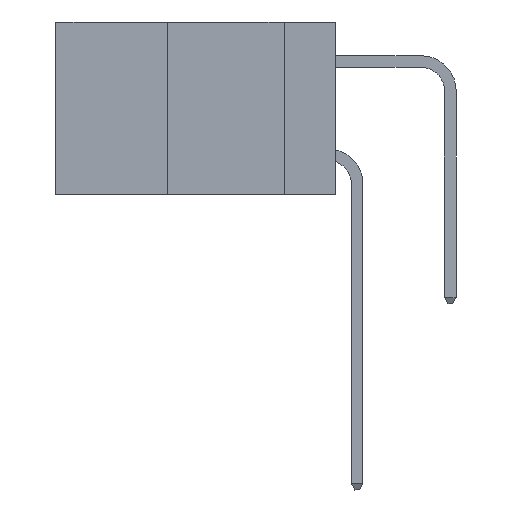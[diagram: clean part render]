
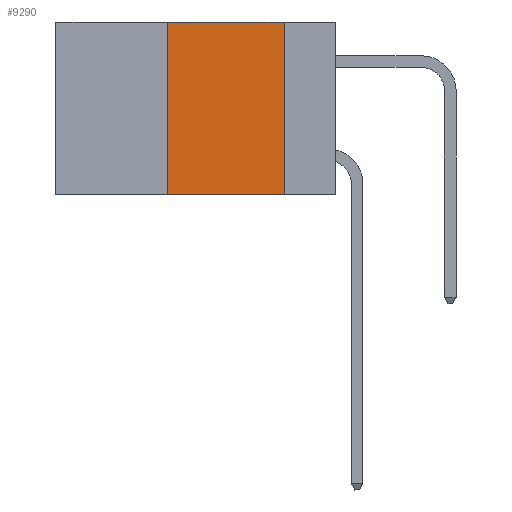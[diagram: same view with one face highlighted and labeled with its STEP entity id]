
A CAD part, left-side view. The second image highlights one B-rep face of the part: STEP entity #9290.
In plain terms, the highlighted planar face has unit normal (-1, 0, 0).
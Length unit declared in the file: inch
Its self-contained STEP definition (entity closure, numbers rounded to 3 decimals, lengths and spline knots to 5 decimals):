
#81 = ORIENTED_EDGE ( 'NONE', *, *, #43969, .F. ) ;
#758 = CARTESIAN_POINT ( 'NONE',  ( 0., 0.36, -0.37 ) ) ;
#1697 = CARTESIAN_POINT ( 'NONE',  ( 0., 0.6, 0. ) ) ;
#3826 = EDGE_CURVE ( 'NONE', #9792, #38395, #30801, .T. ) ;
#5704 = LINE ( 'NONE', #38558, #42767 ) ;
#8348 = CARTESIAN_POINT ( 'NONE',  ( 0., 0.6, -0.37 ) ) ;
#8599 = VECTOR ( 'NONE', #31343, 39.37008 ) ;
#9290 = ADVANCED_FACE ( 'NONE', ( #27947 ), #39263, .F. ) ;
#9792 = VERTEX_POINT ( 'NONE', #758 ) ;
#9889 = CARTESIAN_POINT ( 'NONE',  ( 0., 0.11, 0. ) ) ;
#10367 = ORIENTED_EDGE ( 'NONE', *, *, #3826, .T. ) ;
#10488 = LINE ( 'NONE', #17383, #14253 ) ;
#12723 = CARTESIAN_POINT ( 'NONE',  ( 0., 0.36, 0. ) ) ;
#13116 = VERTEX_POINT ( 'NONE', #9889 ) ;
#14253 = VECTOR ( 'NONE', #28776, 39.37008 ) ;
#14943 = DIRECTION ( 'NONE',  ( 1., 0., 0. ) ) ;
#17383 = CARTESIAN_POINT ( 'NONE',  ( 0., 0.36, 0. ) ) ;
#17480 = EDGE_CURVE ( 'NONE', #41739, #13116, #5704, .T. ) ;
#19195 = EDGE_CURVE ( 'NONE', #9792, #41739, #10488, .T. ) ;
#19458 = EDGE_LOOP ( 'NONE', ( #81, #43037, #34671, #10367 ) ) ;
#25228 = DIRECTION ( 'NONE',  ( 0., -1., 0. ) ) ;
#25357 = DIRECTION ( 'NONE',  ( 0., -1., 0. ) ) ;
#27947 = FACE_OUTER_BOUND ( 'NONE', #19458, .T. ) ;
#28776 = DIRECTION ( 'NONE',  ( 0., 0., 1. ) ) ;
#30145 = LINE ( 'NONE', #31486, #8599 ) ;
#30801 = LINE ( 'NONE', #8348, #38330 ) ;
#31343 = DIRECTION ( 'NONE',  ( 0., 0., -1. ) ) ;
#31486 = CARTESIAN_POINT ( 'NONE',  ( 0., 0.11, 0. ) ) ;
#34671 = ORIENTED_EDGE ( 'NONE', *, *, #19195, .F. ) ;
#38330 = VECTOR ( 'NONE', #25228, 39.37008 ) ;
#38395 = VERTEX_POINT ( 'NONE', #42827 ) ;
#38558 = CARTESIAN_POINT ( 'NONE',  ( 0., 0.6, 0. ) ) ;
#39263 = PLANE ( 'NONE',  #39875 ) ;
#39416 = DIRECTION ( 'NONE',  ( 0., 0., -1. ) ) ;
#39875 = AXIS2_PLACEMENT_3D ( 'NONE', #1697, #14943, #39416 ) ;
#41739 = VERTEX_POINT ( 'NONE', #12723 ) ;
#42767 = VECTOR ( 'NONE', #25357, 39.37008 ) ;
#42827 = CARTESIAN_POINT ( 'NONE',  ( 0., 0.11, -0.37 ) ) ;
#43037 = ORIENTED_EDGE ( 'NONE', *, *, #17480, .F. ) ;
#43969 = EDGE_CURVE ( 'NONE', #13116, #38395, #30145, .T. ) ;
